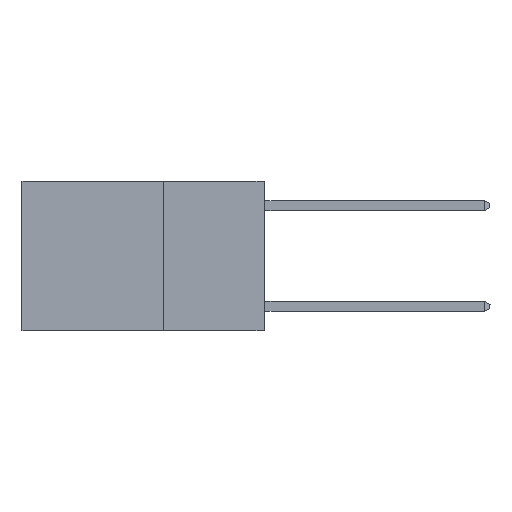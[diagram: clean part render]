
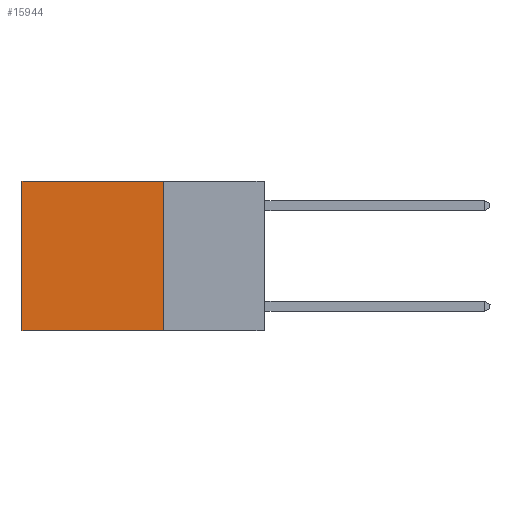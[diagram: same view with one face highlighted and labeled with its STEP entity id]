
A CAD part, left-side view. The second image highlights one B-rep face of the part: STEP entity #15944.
In plain terms, the highlighted planar face has unit normal (-1, 0, 0).
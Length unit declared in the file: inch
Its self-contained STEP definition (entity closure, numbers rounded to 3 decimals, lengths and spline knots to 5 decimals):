
#1130 = VERTEX_POINT ( 'NONE', #16144 ) ;
#1131 = FACE_OUTER_BOUND ( 'NONE', #12606, .T. ) ;
#1381 = DIRECTION ( 'NONE',  ( 0., 0., -1. ) ) ;
#1556 = LINE ( 'NONE', #16108, #16043 ) ;
#1797 = VECTOR ( 'NONE', #8041, 39.37008 ) ;
#2498 = VECTOR ( 'NONE', #5841, 39.37008 ) ;
#2823 = EDGE_CURVE ( 'NONE', #6865, #12757, #11874, .T. ) ;
#2854 = CARTESIAN_POINT ( 'NONE',  ( 0.2625, 0.25, -0.37 ) ) ;
#3514 = AXIS2_PLACEMENT_3D ( 'NONE', #4057, #5483, #14941 ) ;
#4057 = CARTESIAN_POINT ( 'NONE',  ( 0.2625, 0.25, 0. ) ) ;
#4225 = VERTEX_POINT ( 'NONE', #2854 ) ;
#5048 = EDGE_CURVE ( 'NONE', #4225, #12757, #16273, .T. ) ;
#5059 = ORIENTED_EDGE ( 'NONE', *, *, #5048, .F. ) ;
#5483 = DIRECTION ( 'NONE',  ( 1., 0., 0. ) ) ;
#5804 = EDGE_CURVE ( 'NONE', #1130, #4225, #1556, .T. ) ;
#5841 = DIRECTION ( 'NONE',  ( 0., 1., 0. ) ) ;
#6865 = VERTEX_POINT ( 'NONE', #8954 ) ;
#7550 = ORIENTED_EDGE ( 'NONE', *, *, #15475, .T. ) ;
#8041 = DIRECTION ( 'NONE',  ( 0., 1., 0. ) ) ;
#8954 = CARTESIAN_POINT ( 'NONE',  ( 0.2625, 0.6, 0. ) ) ;
#9479 = LINE ( 'NONE', #15287, #2498 ) ;
#11149 = CARTESIAN_POINT ( 'NONE',  ( 0.2625, 0.6, 0. ) ) ;
#11822 = ORIENTED_EDGE ( 'NONE', *, *, #2823, .T. ) ;
#11874 = LINE ( 'NONE', #11149, #14523 ) ;
#12324 = PLANE ( 'NONE',  #3514 ) ;
#12606 = EDGE_LOOP ( 'NONE', ( #11822, #5059, #14594, #7550 ) ) ;
#12757 = VERTEX_POINT ( 'NONE', #14869 ) ;
#13546 = DIRECTION ( 'NONE',  ( 0., 0., -1. ) ) ;
#14523 = VECTOR ( 'NONE', #1381, 39.37008 ) ;
#14594 = ORIENTED_EDGE ( 'NONE', *, *, #5804, .F. ) ;
#14869 = CARTESIAN_POINT ( 'NONE',  ( 0.2625, 0.6, -0.37 ) ) ;
#14941 = DIRECTION ( 'NONE',  ( 0., 0., -1. ) ) ;
#15287 = CARTESIAN_POINT ( 'NONE',  ( 0.2625, 0.25, 0. ) ) ;
#15475 = EDGE_CURVE ( 'NONE', #1130, #6865, #9479, .T. ) ;
#15944 = ADVANCED_FACE ( 'NONE', ( #1131 ), #12324, .F. ) ;
#16043 = VECTOR ( 'NONE', #13546, 39.37008 ) ;
#16108 = CARTESIAN_POINT ( 'NONE',  ( 0.2625, 0.25, 0. ) ) ;
#16144 = CARTESIAN_POINT ( 'NONE',  ( 0.2625, 0.25, 0. ) ) ;
#16273 = LINE ( 'NONE', #17321, #1797 ) ;
#17321 = CARTESIAN_POINT ( 'NONE',  ( 0.2625, 0.25, -0.37 ) ) ;
